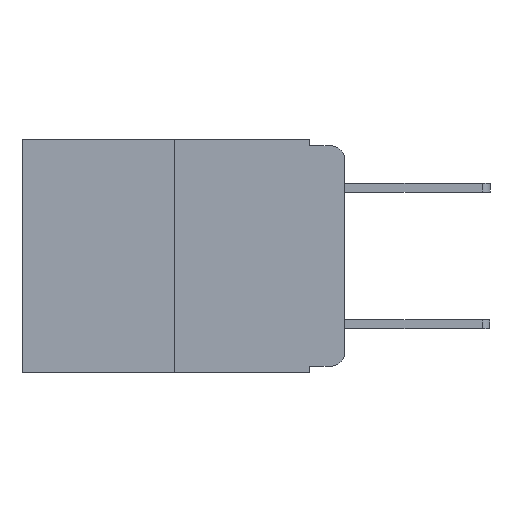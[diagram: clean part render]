
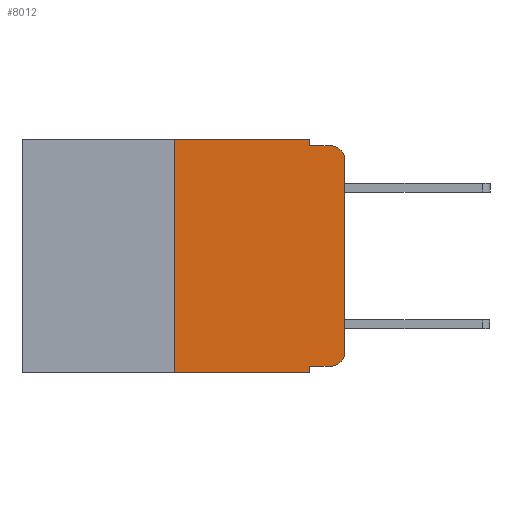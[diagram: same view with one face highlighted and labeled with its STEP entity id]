
A CAD part, left-side view. The second image highlights one B-rep face of the part: STEP entity #8012.
In plain terms, the highlighted planar face has unit normal (-1, 0, 0).
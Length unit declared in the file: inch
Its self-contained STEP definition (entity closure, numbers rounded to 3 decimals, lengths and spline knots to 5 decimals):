
#641 = CARTESIAN_POINT ( 'NONE',  ( 0., 0., -0.313 ) ) ;
#738 = AXIS2_PLACEMENT_3D ( 'NONE', #5074, #14297, #6437 ) ;
#1625 = DIRECTION ( 'NONE',  ( 0., 0., 1. ) ) ;
#2040 = CIRCLE ( 'NONE', #738, 0.02 ) ;
#2408 = CARTESIAN_POINT ( 'NONE',  ( 0., 0.02, -0.03 ) ) ;
#2488 = DIRECTION ( 'NONE',  ( 0., -1., 0. ) ) ;
#2720 = VERTEX_POINT ( 'NONE', #12492 ) ;
#2847 = EDGE_CURVE ( 'NONE', #3557, #16430, #6562, .T. ) ;
#3028 = LINE ( 'NONE', #12730, #9875 ) ;
#3247 = LINE ( 'NONE', #6666, #16890 ) ;
#3331 = DIRECTION ( 'NONE',  ( 0., 0., 1. ) ) ;
#3351 = CARTESIAN_POINT ( 'NONE',  ( 0., 0.051, -0.333 ) ) ;
#3557 = VERTEX_POINT ( 'NONE', #3351 ) ;
#3856 = DIRECTION ( 'NONE',  ( 0., 0., -1. ) ) ;
#3866 = EDGE_LOOP ( 'NONE', ( #15579, #13992, #15945, #12199, #12440, #15736, #17067, #8173, #8349, #16449 ) ) ;
#3983 = AXIS2_PLACEMENT_3D ( 'NONE', #2408, #11915, #3856 ) ;
#4213 = VECTOR ( 'NONE', #13863, 39.37008 ) ;
#4345 = DIRECTION ( 'NONE',  ( 0., 0., -1. ) ) ;
#4519 = EDGE_CURVE ( 'NONE', #3557, #12280, #3247, .T. ) ;
#4662 = CARTESIAN_POINT ( 'NONE',  ( 0., 0.051, 0. ) ) ;
#4835 = CIRCLE ( 'NONE', #3983, 0.02 ) ;
#4934 = VECTOR ( 'NONE', #2488, 39.37008 ) ;
#5074 = CARTESIAN_POINT ( 'NONE',  ( 0., 0.02, -0.313 ) ) ;
#5110 = EDGE_CURVE ( 'NONE', #12670, #16296, #15706, .T. ) ;
#5156 = CARTESIAN_POINT ( 'NONE',  ( 0., 0.25, -0.343 ) ) ;
#5220 = VECTOR ( 'NONE', #1625, 39.37008 ) ;
#5284 = CARTESIAN_POINT ( 'NONE',  ( 0., 0.25, 0. ) ) ;
#5766 = CARTESIAN_POINT ( 'NONE',  ( 0., 0.051, 0. ) ) ;
#5783 = VECTOR ( 'NONE', #9033, 39.37008 ) ;
#6033 = DIRECTION ( 'NONE',  ( 0., 0., -1. ) ) ;
#6133 = VECTOR ( 'NONE', #10764, 39.37008 ) ;
#6437 = DIRECTION ( 'NONE',  ( 0., 0., -1. ) ) ;
#6562 = LINE ( 'NONE', #11229, #6133 ) ;
#6666 = CARTESIAN_POINT ( 'NONE',  ( 0., 0.051, 0. ) ) ;
#6906 = CARTESIAN_POINT ( 'NONE',  ( 0., 0.02, -0.333 ) ) ;
#7009 = VERTEX_POINT ( 'NONE', #5766 ) ;
#7097 = CARTESIAN_POINT ( 'NONE',  ( 0., 0.473, 0. ) ) ;
#7125 = CARTESIAN_POINT ( 'NONE',  ( 0., 0.051, -0.343 ) ) ;
#7877 = LINE ( 'NONE', #12589, #4213 ) ;
#8012 = ADVANCED_FACE ( 'NONE', ( #12998 ), #8419, .F. ) ;
#8013 = CARTESIAN_POINT ( 'NONE',  ( 0., 0.25, 0. ) ) ;
#8173 = ORIENTED_EDGE ( 'NONE', *, *, #4519, .F. ) ;
#8349 = ORIENTED_EDGE ( 'NONE', *, *, #2847, .T. ) ;
#8419 = PLANE ( 'NONE',  #16547 ) ;
#8481 = DIRECTION ( 'NONE',  ( 0., 0., -1. ) ) ;
#9033 = DIRECTION ( 'NONE',  ( 0., -1., 0. ) ) ;
#9345 = CARTESIAN_POINT ( 'NONE',  ( 0., 0.051, -0.01 ) ) ;
#9875 = VECTOR ( 'NONE', #3331, 39.37008 ) ;
#10234 = VERTEX_POINT ( 'NONE', #15284 ) ;
#10417 = VECTOR ( 'NONE', #6033, 39.37008 ) ;
#10764 = DIRECTION ( 'NONE',  ( 0., -1., 0. ) ) ;
#11229 = CARTESIAN_POINT ( 'NONE',  ( 0., 0.051, -0.333 ) ) ;
#11542 = EDGE_CURVE ( 'NONE', #12670, #12280, #7877, .T. ) ;
#11877 = VERTEX_POINT ( 'NONE', #13298 ) ;
#11915 = DIRECTION ( 'NONE',  ( -1., 0., 0. ) ) ;
#12064 = LINE ( 'NONE', #9345, #4934 ) ;
#12199 = ORIENTED_EDGE ( 'NONE', *, *, #15988, .F. ) ;
#12280 = VERTEX_POINT ( 'NONE', #7125 ) ;
#12440 = ORIENTED_EDGE ( 'NONE', *, *, #16758, .F. ) ;
#12454 = LINE ( 'NONE', #16860, #5783 ) ;
#12492 = CARTESIAN_POINT ( 'NONE',  ( 0., 0.02, -0.01 ) ) ;
#12542 = VERTEX_POINT ( 'NONE', #641 ) ;
#12589 = CARTESIAN_POINT ( 'NONE',  ( 0., 0.473, -0.343 ) ) ;
#12670 = VERTEX_POINT ( 'NONE', #5156 ) ;
#12730 = CARTESIAN_POINT ( 'NONE',  ( 0., 0., 0. ) ) ;
#12998 = FACE_OUTER_BOUND ( 'NONE', #3866, .T. ) ;
#13298 = CARTESIAN_POINT ( 'NONE',  ( 0., 0., -0.03 ) ) ;
#13374 = EDGE_CURVE ( 'NONE', #11877, #2720, #4835, .T. ) ;
#13469 = LINE ( 'NONE', #4662, #10417 ) ;
#13863 = DIRECTION ( 'NONE',  ( 0., -1., 0. ) ) ;
#13992 = ORIENTED_EDGE ( 'NONE', *, *, #13374, .T. ) ;
#14297 = DIRECTION ( 'NONE',  ( -1., 0., 0. ) ) ;
#14360 = EDGE_CURVE ( 'NONE', #12542, #11877, #3028, .T. ) ;
#15284 = CARTESIAN_POINT ( 'NONE',  ( 0., 0.051, -0.01 ) ) ;
#15579 = ORIENTED_EDGE ( 'NONE', *, *, #14360, .T. ) ;
#15706 = LINE ( 'NONE', #5284, #5220 ) ;
#15736 = ORIENTED_EDGE ( 'NONE', *, *, #5110, .F. ) ;
#15945 = ORIENTED_EDGE ( 'NONE', *, *, #16297, .F. ) ;
#15988 = EDGE_CURVE ( 'NONE', #7009, #10234, #13469, .T. ) ;
#16195 = DIRECTION ( 'NONE',  ( 1., 0., 0. ) ) ;
#16296 = VERTEX_POINT ( 'NONE', #8013 ) ;
#16297 = EDGE_CURVE ( 'NONE', #10234, #2720, #12064, .T. ) ;
#16430 = VERTEX_POINT ( 'NONE', #6906 ) ;
#16449 = ORIENTED_EDGE ( 'NONE', *, *, #16744, .T. ) ;
#16547 = AXIS2_PLACEMENT_3D ( 'NONE', #7097, #16195, #8481 ) ;
#16744 = EDGE_CURVE ( 'NONE', #16430, #12542, #2040, .T. ) ;
#16758 = EDGE_CURVE ( 'NONE', #16296, #7009, #12454, .T. ) ;
#16860 = CARTESIAN_POINT ( 'NONE',  ( 0., 0.473, 0. ) ) ;
#16890 = VECTOR ( 'NONE', #4345, 39.37008 ) ;
#17067 = ORIENTED_EDGE ( 'NONE', *, *, #11542, .T. ) ;
